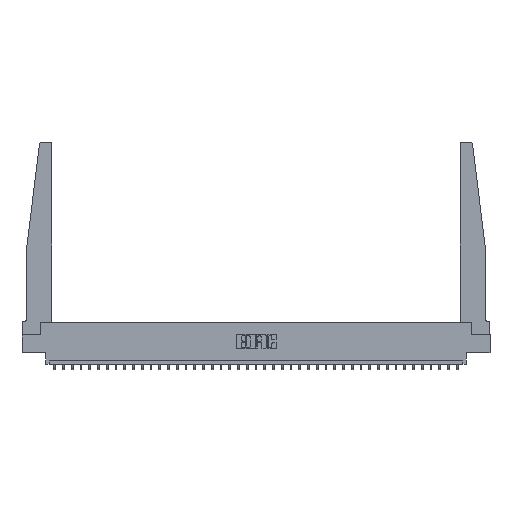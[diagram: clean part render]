
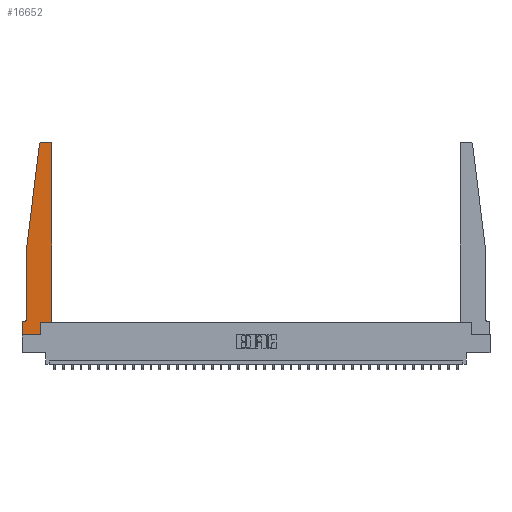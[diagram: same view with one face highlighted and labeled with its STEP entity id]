
A CAD part, top view. The second image highlights one B-rep face of the part: STEP entity #16652.
In plain terms, the highlighted planar face has unit normal (0, 0, 1).
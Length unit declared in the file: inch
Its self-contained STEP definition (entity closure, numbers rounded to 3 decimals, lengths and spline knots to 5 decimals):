
#642 = LINE ( 'NONE', #26235, #2256 ) ;
#2009 = CARTESIAN_POINT ( 'NONE',  ( 0.27653, 2.72, 0.37 ) ) ;
#2256 = VECTOR ( 'NONE', #13390, 39.37008 ) ;
#2258 = EDGE_LOOP ( 'NONE', ( #14752, #27654, #32884, #17598, #5382, #23645, #15144, #19611, #6611, #17219, #4965, #9479 ) ) ;
#2903 = DIRECTION ( 'NONE',  ( 0., 0., -1. ) ) ;
#3201 = CARTESIAN_POINT ( 'NONE',  ( 0.24675, 2.72367, 0.37 ) ) ;
#4146 = VECTOR ( 'NONE', #9150, 39.37008 ) ;
#4473 = VECTOR ( 'NONE', #16469, 39.37008 ) ;
#4595 = DIRECTION ( 'NONE',  ( 1., 0., 0. ) ) ;
#4965 = ORIENTED_EDGE ( 'NONE', *, *, #20306, .T. ) ;
#5135 = EDGE_CURVE ( 'NONE', #8403, #10657, #9100, .T. ) ;
#5382 = ORIENTED_EDGE ( 'NONE', *, *, #5135, .T. ) ;
#6308 = VECTOR ( 'NONE', #28385, 39.37008 ) ;
#6611 = ORIENTED_EDGE ( 'NONE', *, *, #12738, .T. ) ;
#7331 = CIRCLE ( 'NONE', #26603, 0.03 ) ;
#7542 = LINE ( 'NONE', #19295, #28138 ) ;
#7748 = EDGE_CURVE ( 'NONE', #13106, #22150, #17402, .T. ) ;
#8403 = VERTEX_POINT ( 'NONE', #11580 ) ;
#9100 = CIRCLE ( 'NONE', #9300, 0.05 ) ;
#9150 = DIRECTION ( 'NONE',  ( -1., 0., 0. ) ) ;
#9180 = VECTOR ( 'NONE', #30276, 39.37008 ) ;
#9300 = AXIS2_PLACEMENT_3D ( 'NONE', #18492, #2903, #21075 ) ;
#9479 = ORIENTED_EDGE ( 'NONE', *, *, #29980, .T. ) ;
#9951 = EDGE_CURVE ( 'NONE', #21287, #13091, #28545, .T. ) ;
#10657 = VERTEX_POINT ( 'NONE', #25785 ) ;
#10825 = VECTOR ( 'NONE', #11175, 39.37008 ) ;
#11175 = DIRECTION ( 'NONE',  ( 1., 0., 0. ) ) ;
#11284 = PLANE ( 'NONE',  #19168 ) ;
#11417 = LINE ( 'NONE', #24146, #4473 ) ;
#11580 = CARTESIAN_POINT ( 'NONE',  ( 0.065, 0.2375, 0.37 ) ) ;
#11736 = VERTEX_POINT ( 'NONE', #30154 ) ;
#11740 = CARTESIAN_POINT ( 'NONE',  ( 0.395, 2.72, 0.37 ) ) ;
#12067 = CARTESIAN_POINT ( 'NONE',  ( 0.425, 0.18, 0.37 ) ) ;
#12629 = FACE_OUTER_BOUND ( 'NONE', #2258, .T. ) ;
#12738 = EDGE_CURVE ( 'NONE', #16674, #11736, #11417, .T. ) ;
#12975 = CARTESIAN_POINT ( 'NONE',  ( 0.25, 2.75, 0.37 ) ) ;
#13091 = VERTEX_POINT ( 'NONE', #30631 ) ;
#13106 = VERTEX_POINT ( 'NONE', #33234 ) ;
#13111 = VECTOR ( 'NONE', #27853, 39.37008 ) ;
#13176 = CARTESIAN_POINT ( 'NONE',  ( 0.425, 2.72, 0.37 ) ) ;
#13390 = DIRECTION ( 'NONE',  ( -0.122, -0.992, 0. ) ) ;
#13785 = LINE ( 'NONE', #14844, #9180 ) ;
#13889 = DIRECTION ( 'NONE',  ( 0., 0., 1. ) ) ;
#13911 = LINE ( 'NONE', #20121, #13111 ) ;
#14336 = DIRECTION ( 'NONE',  ( 1., 0., 0. ) ) ;
#14752 = ORIENTED_EDGE ( 'NONE', *, *, #9951, .T. ) ;
#14844 = CARTESIAN_POINT ( 'NONE',  ( 0.065, 1.25, 0.37 ) ) ;
#15144 = ORIENTED_EDGE ( 'NONE', *, *, #7748, .T. ) ;
#15278 = CARTESIAN_POINT ( 'NONE',  ( 0.395, 2.75, 0.37 ) ) ;
#16077 = CARTESIAN_POINT ( 'NONE',  ( 0., 0., 0.37 ) ) ;
#16469 = DIRECTION ( 'NONE',  ( 0., 1., 0. ) ) ;
#16489 = CARTESIAN_POINT ( 'NONE',  ( 0.2605, 0., 0.37 ) ) ;
#16652 = ADVANCED_FACE ( 'NONE', ( #12629 ), #11284, .T. ) ;
#16674 = VERTEX_POINT ( 'NONE', #16489 ) ;
#17219 = ORIENTED_EDGE ( 'NONE', *, *, #27184, .T. ) ;
#17402 = LINE ( 'NONE', #16077, #24236 ) ;
#17442 = CARTESIAN_POINT ( 'NONE',  ( 0.065, 1.25, 0.37 ) ) ;
#17598 = ORIENTED_EDGE ( 'NONE', *, *, #28933, .T. ) ;
#17984 = LINE ( 'NONE', #27190, #4146 ) ;
#18492 = CARTESIAN_POINT ( 'NONE',  ( 0.015, 0.2375, 0.37 ) ) ;
#18689 = AXIS2_PLACEMENT_3D ( 'NONE', #11740, #29747, #14336 ) ;
#19168 = AXIS2_PLACEMENT_3D ( 'NONE', #29295, #13889, #31902 ) ;
#19295 = CARTESIAN_POINT ( 'NONE',  ( 0.425, 0.18, 0.37 ) ) ;
#19611 = ORIENTED_EDGE ( 'NONE', *, *, #19722, .T. ) ;
#19722 = EDGE_CURVE ( 'NONE', #22150, #16674, #26176, .T. ) ;
#20121 = CARTESIAN_POINT ( 'NONE',  ( 0.425, 0.18, 0.37 ) ) ;
#20175 = DIRECTION ( 'NONE',  ( 0., 0., 1. ) ) ;
#20306 = EDGE_CURVE ( 'NONE', #24821, #25112, #7542, .T. ) ;
#21075 = DIRECTION ( 'NONE',  ( -1., 0., 0. ) ) ;
#21287 = VERTEX_POINT ( 'NONE', #15278 ) ;
#21526 = VERTEX_POINT ( 'NONE', #3201 ) ;
#22150 = VERTEX_POINT ( 'NONE', #31316 ) ;
#22623 = CIRCLE ( 'NONE', #18689, 0.03 ) ;
#23645 = ORIENTED_EDGE ( 'NONE', *, *, #27046, .T. ) ;
#24042 = CARTESIAN_POINT ( 'NONE',  ( 0., 0., 0.37 ) ) ;
#24146 = CARTESIAN_POINT ( 'NONE',  ( 0.2605, 0.18, 0.37 ) ) ;
#24202 = VERTEX_POINT ( 'NONE', #17442 ) ;
#24236 = VECTOR ( 'NONE', #28906, 39.37008 ) ;
#24485 = DIRECTION ( 'NONE',  ( 0., 1., 0. ) ) ;
#24821 = VERTEX_POINT ( 'NONE', #12067 ) ;
#25112 = VERTEX_POINT ( 'NONE', #13176 ) ;
#25785 = CARTESIAN_POINT ( 'NONE',  ( 0.015, 0.1875, 0.37 ) ) ;
#26148 = EDGE_CURVE ( 'NONE', #21526, #24202, #642, .T. ) ;
#26176 = LINE ( 'NONE', #24042, #10825 ) ;
#26235 = CARTESIAN_POINT ( 'NONE',  ( 0.065, 1.25, 0.37 ) ) ;
#26603 = AXIS2_PLACEMENT_3D ( 'NONE', #2009, #20175, #4595 ) ;
#27046 = EDGE_CURVE ( 'NONE', #10657, #13106, #17984, .T. ) ;
#27184 = EDGE_CURVE ( 'NONE', #11736, #24821, #13911, .T. ) ;
#27190 = CARTESIAN_POINT ( 'NONE',  ( 0.065, 0.1875, 0.37 ) ) ;
#27654 = ORIENTED_EDGE ( 'NONE', *, *, #28257, .T. ) ;
#27853 = DIRECTION ( 'NONE',  ( 1., 0., 0. ) ) ;
#28138 = VECTOR ( 'NONE', #24485, 39.37008 ) ;
#28257 = EDGE_CURVE ( 'NONE', #13091, #21526, #7331, .T. ) ;
#28385 = DIRECTION ( 'NONE',  ( -1., 0., 0. ) ) ;
#28545 = LINE ( 'NONE', #12975, #6308 ) ;
#28906 = DIRECTION ( 'NONE',  ( 0., -1., 0. ) ) ;
#28933 = EDGE_CURVE ( 'NONE', #24202, #8403, #13785, .T. ) ;
#29295 = CARTESIAN_POINT ( 'NONE',  ( 0., 0.1875, 0.37 ) ) ;
#29747 = DIRECTION ( 'NONE',  ( 0., 0., 1. ) ) ;
#29980 = EDGE_CURVE ( 'NONE', #25112, #21287, #22623, .T. ) ;
#30154 = CARTESIAN_POINT ( 'NONE',  ( 0.2605, 0.18, 0.37 ) ) ;
#30276 = DIRECTION ( 'NONE',  ( 0., -1., 0. ) ) ;
#30631 = CARTESIAN_POINT ( 'NONE',  ( 0.27653, 2.75, 0.37 ) ) ;
#31316 = CARTESIAN_POINT ( 'NONE',  ( 0., 0., 0.37 ) ) ;
#31902 = DIRECTION ( 'NONE',  ( 1., 0., 0. ) ) ;
#32884 = ORIENTED_EDGE ( 'NONE', *, *, #26148, .T. ) ;
#33234 = CARTESIAN_POINT ( 'NONE',  ( 0., 0.1875, 0.37 ) ) ;
